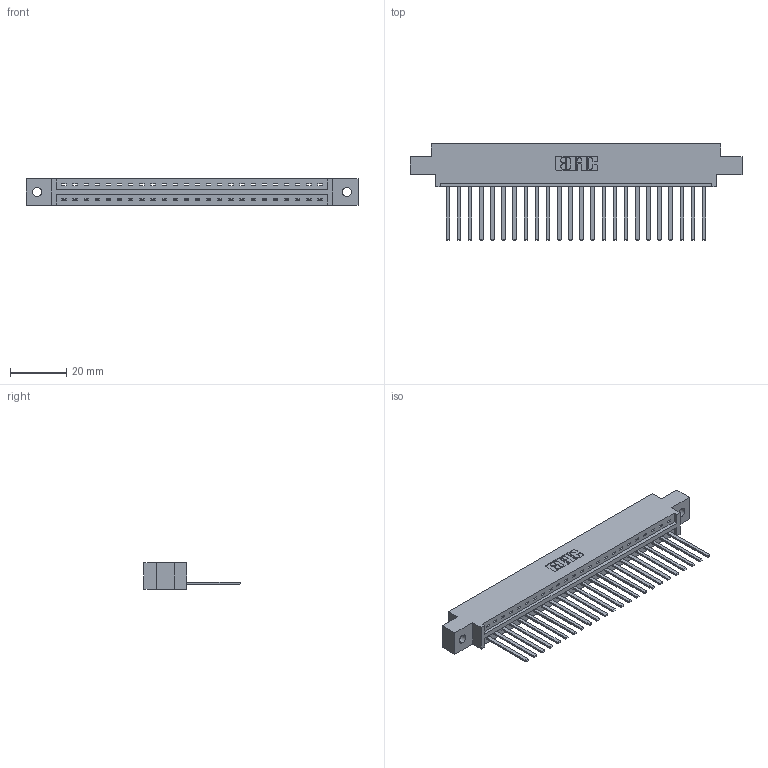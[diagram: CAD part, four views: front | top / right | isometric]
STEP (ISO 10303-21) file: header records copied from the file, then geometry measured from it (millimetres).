
FILE_DESCRIPTION (( 'STEP AP203' ), '1' );
FILE_NAME ('337-024-544-602.STEP', '2019-09-30T16:07:52', ( '' ), ( '' ), 'SwSTEP 2.0', 'SolidWorks 2016', '' );
FILE_SCHEMA (( 'CONFIG_CONTROL_DESIGN' ));
Length unit declared in the file: inch
Products named in the file (3): 345-292-001_345-293-144; 337-024-544-602; 337 Part_0.170 Offset - 0.128 Dia
Assembly tree (25 placements, depth 2):
  337-024-544-602
    337 Part_0.170 Offset - 0.128 Dia
    345-292-001_345-293-144  x24
Bounding box: 118.11 x 34.3 x 9.4 mm (x, y, z)
Volume: 12174.1 mm3; surface area: 13221.1 mm2
Topology: 25 solids, 25 shells, 1462 faces, 4403 edges, 2902 vertices
Faces by surface type: plane 1082, cylinder 380
Entity records: 20119 total; most frequent: CARTESIAN_POINT 3510, ORIENTED_EDGE 3470, DIRECTION 2987, EDGE_CURVE 1735, VECTOR 1611, LINE 1611, VERTEX_POINT 1154, AXIS2_PLACEMENT_3D 688
